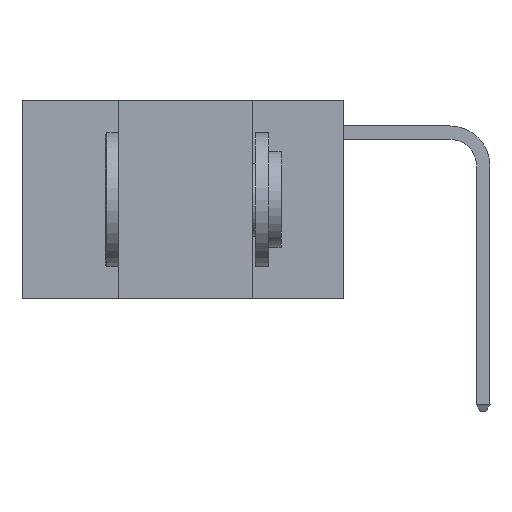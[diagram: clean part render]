
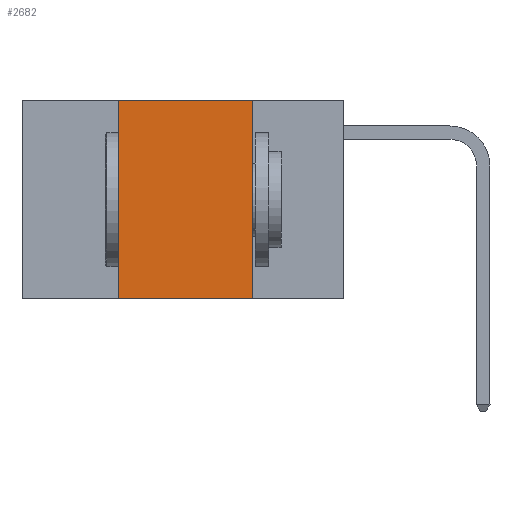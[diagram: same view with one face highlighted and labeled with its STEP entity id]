
A CAD part, left-side view. The second image highlights one B-rep face of the part: STEP entity #2682.
In plain terms, the highlighted planar face has unit normal (-1, 0, 0).
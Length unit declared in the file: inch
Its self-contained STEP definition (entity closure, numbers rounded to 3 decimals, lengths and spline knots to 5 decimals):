
#1972 = VERTEX_POINT ( 'NONE', #18133 ) ;
#2676 = DIRECTION ( 'NONE',  ( 0., -1., 0. ) ) ;
#2682 = ADVANCED_FACE ( 'NONE', ( #15148 ), #12527, .F. ) ;
#2716 = LINE ( 'NONE', #19765, #13511 ) ;
#2816 = AXIS2_PLACEMENT_3D ( 'NONE', #4610, #13078, #21543 ) ;
#2992 = CARTESIAN_POINT ( 'NONE',  ( 0., 0.17, -0.37 ) ) ;
#4610 = CARTESIAN_POINT ( 'NONE',  ( 0., 0.6, 0. ) ) ;
#4680 = ORIENTED_EDGE ( 'NONE', *, *, #15810, .F. ) ;
#5120 = DIRECTION ( 'NONE',  ( 0., 0., 1. ) ) ;
#5755 = VECTOR ( 'NONE', #2676, 39.37008 ) ;
#6670 = CARTESIAN_POINT ( 'NONE',  ( 0., 0.6, -0.37 ) ) ;
#7747 = CARTESIAN_POINT ( 'NONE',  ( 0., 0.42, 0. ) ) ;
#8645 = EDGE_CURVE ( 'NONE', #1972, #12342, #15675, .T. ) ;
#8744 = LINE ( 'NONE', #6670, #5755 ) ;
#10825 = VERTEX_POINT ( 'NONE', #2992 ) ;
#11283 = VECTOR ( 'NONE', #5120, 39.37008 ) ;
#12327 = EDGE_LOOP ( 'NONE', ( #4680, #26364, #25605, #25476 ) ) ;
#12342 = VERTEX_POINT ( 'NONE', #14638 ) ;
#12527 = PLANE ( 'NONE',  #2816 ) ;
#12834 = VECTOR ( 'NONE', #24581, 39.37008 ) ;
#13078 = DIRECTION ( 'NONE',  ( 1., 0., 0. ) ) ;
#13511 = VECTOR ( 'NONE', #17689, 39.37008 ) ;
#14628 = CARTESIAN_POINT ( 'NONE',  ( 0., 0.17, 0. ) ) ;
#14638 = CARTESIAN_POINT ( 'NONE',  ( 0., 0.42, 0. ) ) ;
#15148 = FACE_OUTER_BOUND ( 'NONE', #12327, .T. ) ;
#15675 = LINE ( 'NONE', #7747, #11283 ) ;
#15759 = EDGE_CURVE ( 'NONE', #1972, #10825, #8744, .T. ) ;
#15810 = EDGE_CURVE ( 'NONE', #26227, #10825, #16106, .T. ) ;
#16106 = LINE ( 'NONE', #26648, #12834 ) ;
#17689 = DIRECTION ( 'NONE',  ( 0., -1., 0. ) ) ;
#18133 = CARTESIAN_POINT ( 'NONE',  ( 0., 0.42, -0.37 ) ) ;
#19765 = CARTESIAN_POINT ( 'NONE',  ( 0., 0.6, 0. ) ) ;
#21543 = DIRECTION ( 'NONE',  ( 0., 0., -1. ) ) ;
#24009 = EDGE_CURVE ( 'NONE', #12342, #26227, #2716, .T. ) ;
#24581 = DIRECTION ( 'NONE',  ( 0., 0., -1. ) ) ;
#25476 = ORIENTED_EDGE ( 'NONE', *, *, #15759, .T. ) ;
#25605 = ORIENTED_EDGE ( 'NONE', *, *, #8645, .F. ) ;
#26227 = VERTEX_POINT ( 'NONE', #14628 ) ;
#26364 = ORIENTED_EDGE ( 'NONE', *, *, #24009, .F. ) ;
#26648 = CARTESIAN_POINT ( 'NONE',  ( 0., 0.17, 0. ) ) ;
